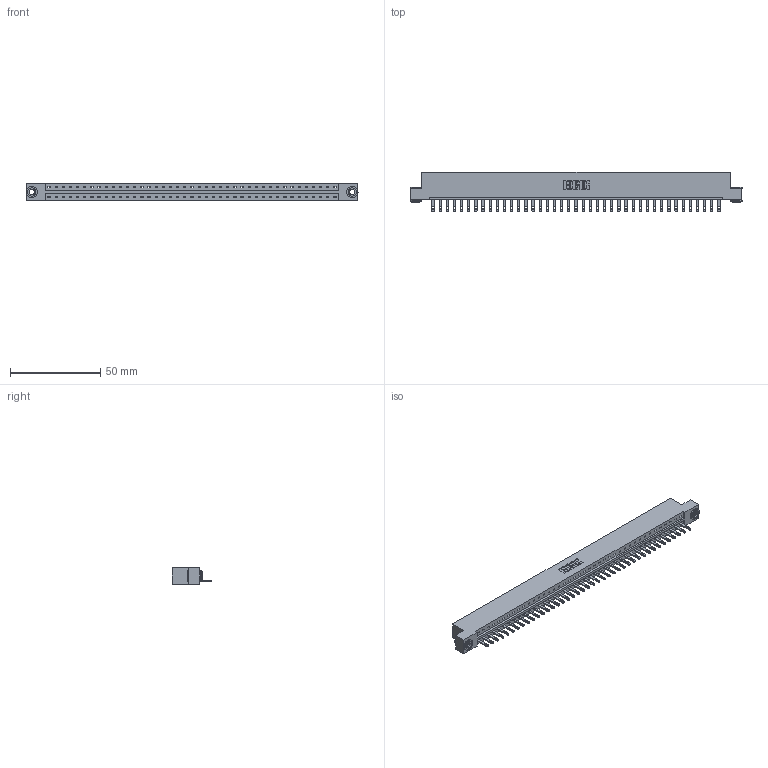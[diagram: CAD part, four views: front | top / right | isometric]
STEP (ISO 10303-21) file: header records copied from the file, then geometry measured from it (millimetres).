
FILE_DESCRIPTION (( 'STEP AP203' ), '1' );
FILE_NAME ('333-041-500-103.STEP', '2018-08-03T15:02:54', ( '' ), ( '' ), 'SwSTEP 2.0', 'SolidWorks 2016', '' );
FILE_SCHEMA (( 'CONFIG_CONTROL_DESIGN' ));
Length unit declared in the file: inch
Products named in the file (4): 345-250-002_345-250-002-102; 333-041-500-103; 333 Part_Flush - .156 Dia - TH; 345-292-001_345-293-100
Assembly tree (44 placements, depth 2):
  333-041-500-103
    333 Part_Flush - .156 Dia - TH
    345-292-001_345-293-100  x41
    345-250-002_345-250-002-102  x2
Bounding box: 184 x 21.85 x 9.4 mm (x, y, z)
Volume: 18551.5 mm3; surface area: 20393.1 mm2
Topology: 44 solids, 44 shells, 2366 faces, 7275 edges, 4846 vertices
Faces by surface type: plane 1556, cylinder 802, cone 8
Entity records: 25774 total; most frequent: CARTESIAN_POINT 4424, ORIENTED_EDGE 4394, DIRECTION 3769, EDGE_CURVE 2197, VECTOR 2041, LINE 2041, VERTEX_POINT 1462, AXIS2_PLACEMENT_3D 864
